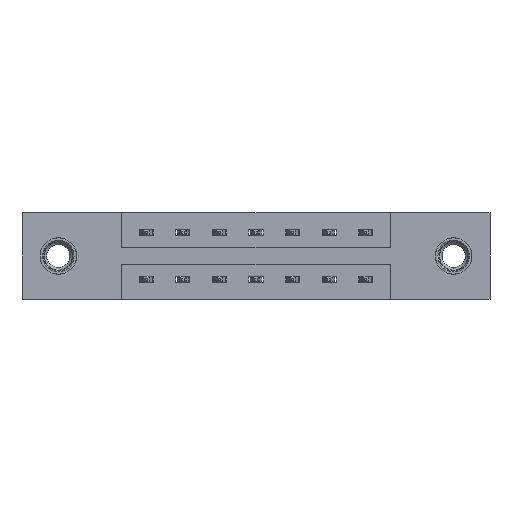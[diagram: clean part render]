
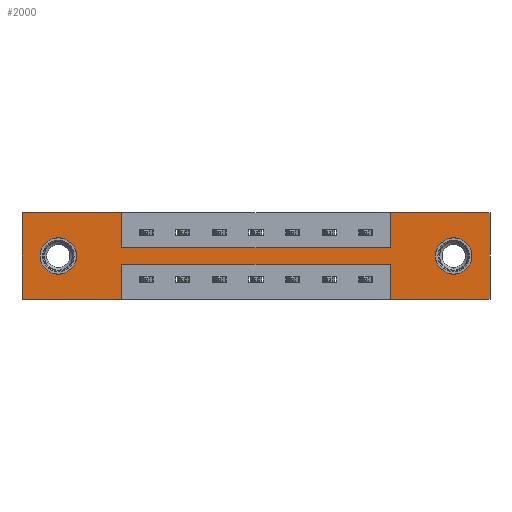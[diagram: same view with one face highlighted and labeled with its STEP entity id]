
A CAD part, front view. The second image highlights one B-rep face of the part: STEP entity #2000.
In plain terms, the highlighted planar face has unit normal (0, -1, 0).
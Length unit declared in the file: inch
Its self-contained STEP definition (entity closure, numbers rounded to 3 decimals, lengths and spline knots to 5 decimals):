
#55 = CIRCLE ( 'NONE', #7593, 0.078 ) ;
#104 = CARTESIAN_POINT ( 'NONE',  ( 1.573, 0., -0.37 ) ) ;
#157 = VECTOR ( 'NONE', #338, 39.37008 ) ;
#312 = DIRECTION ( 'NONE',  ( -1., 0., 0. ) ) ;
#338 = DIRECTION ( 'NONE',  ( 0., 0., -1. ) ) ;
#471 = LINE ( 'NONE', #9917, #2218 ) ;
#537 = CARTESIAN_POINT ( 'NONE',  ( 0., 0., 0. ) ) ;
#622 = VERTEX_POINT ( 'NONE', #3019 ) ;
#650 = DIRECTION ( 'NONE',  ( 0., 1., 0. ) ) ;
#670 = VERTEX_POINT ( 'NONE', #10008 ) ;
#766 = ORIENTED_EDGE ( 'NONE', *, *, #3446, .F. ) ;
#827 = CARTESIAN_POINT ( 'NONE',  ( 0.425, 0., -0.22 ) ) ;
#854 = DIRECTION ( 'NONE',  ( 0., 0., 1. ) ) ;
#955 = VECTOR ( 'NONE', #9980, 39.37008 ) ;
#989 = LINE ( 'NONE', #8020, #9770 ) ;
#1223 = PLANE ( 'NONE',  #6066 ) ;
#1241 = LINE ( 'NONE', #2025, #4396 ) ;
#1275 = LINE ( 'NONE', #104, #6549 ) ;
#1398 = LINE ( 'NONE', #1967, #10052 ) ;
#1524 = DIRECTION ( 'NONE',  ( 0., 1., 0. ) ) ;
#1529 = AXIS2_PLACEMENT_3D ( 'NONE', #5044, #1524, #4934 ) ;
#1532 = VERTEX_POINT ( 'NONE', #7224 ) ;
#1726 = ORIENTED_EDGE ( 'NONE', *, *, #8348, .F. ) ;
#1783 = CIRCLE ( 'NONE', #11081, 0.078 ) ;
#1812 = FACE_BOUND ( 'NONE', #8719, .T. ) ;
#1815 = DIRECTION ( 'NONE',  ( 0., 0., 1. ) ) ;
#1873 = EDGE_CURVE ( 'NONE', #10824, #5733, #471, .T. ) ;
#1967 = CARTESIAN_POINT ( 'NONE',  ( 0.425, 0., -0.22 ) ) ;
#1980 = VECTOR ( 'NONE', #2939, 39.37008 ) ;
#2000 = ADVANCED_FACE ( 'NONE', ( #6968, #1812, #3313 ), #1223, .T. ) ;
#2010 = DIRECTION ( 'NONE',  ( 0., 0., -1. ) ) ;
#2025 = CARTESIAN_POINT ( 'NONE',  ( 0., 0., 0. ) ) ;
#2090 = ORIENTED_EDGE ( 'NONE', *, *, #8855, .F. ) ;
#2108 = CARTESIAN_POINT ( 'NONE',  ( 1.573, 0., -0.15 ) ) ;
#2112 = VERTEX_POINT ( 'NONE', #827 ) ;
#2218 = VECTOR ( 'NONE', #7230, 39.37008 ) ;
#2241 = VERTEX_POINT ( 'NONE', #7441 ) ;
#2256 = CARTESIAN_POINT ( 'NONE',  ( 0.155, 0., -0.185 ) ) ;
#2278 = ORIENTED_EDGE ( 'NONE', *, *, #1873, .F. ) ;
#2280 = DIRECTION ( 'NONE',  ( 0., 0., -1. ) ) ;
#2353 = DIRECTION ( 'NONE',  ( 0., 0., 1. ) ) ;
#2492 = CARTESIAN_POINT ( 'NONE',  ( 0., 0., 0. ) ) ;
#2566 = DIRECTION ( 'NONE',  ( 1., 0., 0. ) ) ;
#2665 = CARTESIAN_POINT ( 'NONE',  ( 0.425, 0., -0.15 ) ) ;
#2847 = ORIENTED_EDGE ( 'NONE', *, *, #11093, .F. ) ;
#2856 = CARTESIAN_POINT ( 'NONE',  ( 0., 0., -0.37 ) ) ;
#2877 = DIRECTION ( 'NONE',  ( 0., 0., -1. ) ) ;
#2923 = DIRECTION ( 'NONE',  ( -1., 0., 0. ) ) ;
#2928 = EDGE_CURVE ( 'NONE', #670, #7029, #5459, .T. ) ;
#2939 = DIRECTION ( 'NONE',  ( 0., 0., -1. ) ) ;
#3000 = ORIENTED_EDGE ( 'NONE', *, *, #4645, .F. ) ;
#3019 = CARTESIAN_POINT ( 'NONE',  ( 0.425, 0., -0.37 ) ) ;
#3028 = EDGE_CURVE ( 'NONE', #10670, #10953, #11077, .T. ) ;
#3039 = AXIS2_PLACEMENT_3D ( 'NONE', #4877, #10363, #854 ) ;
#3173 = VERTEX_POINT ( 'NONE', #9330 ) ;
#3174 = CARTESIAN_POINT ( 'NONE',  ( 1.843, 0., -0.185 ) ) ;
#3216 = DIRECTION ( 'NONE',  ( 0., 0., 1. ) ) ;
#3248 = LINE ( 'NONE', #2492, #7688 ) ;
#3313 = FACE_OUTER_BOUND ( 'NONE', #5036, .T. ) ;
#3354 = CARTESIAN_POINT ( 'NONE',  ( 1.573, 0., 0. ) ) ;
#3416 = ORIENTED_EDGE ( 'NONE', *, *, #3631, .T. ) ;
#3446 = EDGE_CURVE ( 'NONE', #2112, #622, #5840, .T. ) ;
#3631 = EDGE_CURVE ( 'NONE', #10953, #10670, #1783, .T. ) ;
#3747 = ORIENTED_EDGE ( 'NONE', *, *, #2928, .F. ) ;
#4039 = EDGE_CURVE ( 'NONE', #4281, #10824, #8648, .T. ) ;
#4068 = VERTEX_POINT ( 'NONE', #5375 ) ;
#4095 = CARTESIAN_POINT ( 'NONE',  ( 1.843, 0., -0.263 ) ) ;
#4101 = ORIENTED_EDGE ( 'NONE', *, *, #10692, .T. ) ;
#4281 = VERTEX_POINT ( 'NONE', #9925 ) ;
#4396 = VECTOR ( 'NONE', #5483, 39.37008 ) ;
#4645 = EDGE_CURVE ( 'NONE', #4068, #1532, #6584, .T. ) ;
#4877 = CARTESIAN_POINT ( 'NONE',  ( 0.155, 0., -0.185 ) ) ;
#4897 = VECTOR ( 'NONE', #2353, 39.37008 ) ;
#4934 = DIRECTION ( 'NONE',  ( 0., 0., -1. ) ) ;
#4940 = VERTEX_POINT ( 'NONE', #10927 ) ;
#5036 = EDGE_LOOP ( 'NONE', ( #766, #5313, #8299, #7612, #3000, #2090, #1726, #2278, #10695, #2847, #3747, #10406 ) ) ;
#5044 = CARTESIAN_POINT ( 'NONE',  ( 1.843, 0., -0.185 ) ) ;
#5313 = ORIENTED_EDGE ( 'NONE', *, *, #6135, .F. ) ;
#5375 = CARTESIAN_POINT ( 'NONE',  ( 1.998, 0., 0. ) ) ;
#5435 = EDGE_LOOP ( 'NONE', ( #5589, #3416 ) ) ;
#5459 = LINE ( 'NONE', #537, #7866 ) ;
#5483 = DIRECTION ( 'NONE',  ( 1., 0., 0. ) ) ;
#5589 = ORIENTED_EDGE ( 'NONE', *, *, #3028, .T. ) ;
#5645 = DIRECTION ( 'NONE',  ( 0., 0., 1. ) ) ;
#5733 = VERTEX_POINT ( 'NONE', #2108 ) ;
#5840 = LINE ( 'NONE', #8085, #157 ) ;
#5919 = EDGE_CURVE ( 'NONE', #6405, #4940, #1275, .T. ) ;
#5978 = CARTESIAN_POINT ( 'NONE',  ( 1.573, 0., -0.37 ) ) ;
#6066 = AXIS2_PLACEMENT_3D ( 'NONE', #8647, #7202, #2010 ) ;
#6135 = EDGE_CURVE ( 'NONE', #4940, #2112, #1398, .T. ) ;
#6215 = CARTESIAN_POINT ( 'NONE',  ( 0., 0., 0. ) ) ;
#6286 = EDGE_CURVE ( 'NONE', #7742, #2241, #55, .T. ) ;
#6299 = CARTESIAN_POINT ( 'NONE',  ( 0.425, 0., 0. ) ) ;
#6377 = VECTOR ( 'NONE', #2877, 39.37008 ) ;
#6382 = ORIENTED_EDGE ( 'NONE', *, *, #6286, .T. ) ;
#6405 = VERTEX_POINT ( 'NONE', #5978 ) ;
#6549 = VECTOR ( 'NONE', #1815, 39.37008 ) ;
#6584 = LINE ( 'NONE', #10542, #1980 ) ;
#6968 = FACE_BOUND ( 'NONE', #5435, .T. ) ;
#7029 = VERTEX_POINT ( 'NONE', #6215 ) ;
#7202 = DIRECTION ( 'NONE',  ( 0., -1., 0. ) ) ;
#7224 = CARTESIAN_POINT ( 'NONE',  ( 1.998, 0., -0.37 ) ) ;
#7230 = DIRECTION ( 'NONE',  ( 1., 0., 0. ) ) ;
#7338 = CIRCLE ( 'NONE', #3039, 0.078 ) ;
#7441 = CARTESIAN_POINT ( 'NONE',  ( 0.155, 0., -0.263 ) ) ;
#7593 = AXIS2_PLACEMENT_3D ( 'NONE', #2256, #650, #3216 ) ;
#7612 = ORIENTED_EDGE ( 'NONE', *, *, #11122, .F. ) ;
#7688 = VECTOR ( 'NONE', #2566, 39.37008 ) ;
#7742 = VERTEX_POINT ( 'NONE', #10509 ) ;
#7866 = VECTOR ( 'NONE', #5645, 39.37008 ) ;
#8020 = CARTESIAN_POINT ( 'NONE',  ( 0., 0., -0.37 ) ) ;
#8085 = CARTESIAN_POINT ( 'NONE',  ( 0.425, 0., -0.37 ) ) ;
#8299 = ORIENTED_EDGE ( 'NONE', *, *, #5919, .F. ) ;
#8348 = EDGE_CURVE ( 'NONE', #5733, #3173, #9462, .T. ) ;
#8558 = EDGE_CURVE ( 'NONE', #622, #670, #9021, .T. ) ;
#8647 = CARTESIAN_POINT ( 'NONE',  ( 0., 0., -0.37 ) ) ;
#8648 = LINE ( 'NONE', #6299, #6377 ) ;
#8719 = EDGE_LOOP ( 'NONE', ( #6382, #4101 ) ) ;
#8855 = EDGE_CURVE ( 'NONE', #3173, #4068, #3248, .T. ) ;
#9021 = LINE ( 'NONE', #2856, #955 ) ;
#9330 = CARTESIAN_POINT ( 'NONE',  ( 1.573, 0., 0. ) ) ;
#9462 = LINE ( 'NONE', #3354, #4897 ) ;
#9770 = VECTOR ( 'NONE', #2923, 39.37008 ) ;
#9917 = CARTESIAN_POINT ( 'NONE',  ( 0.425, 0., -0.15 ) ) ;
#9925 = CARTESIAN_POINT ( 'NONE',  ( 0.425, 0., 0. ) ) ;
#9939 = DIRECTION ( 'NONE',  ( 0., 1., 0. ) ) ;
#9980 = DIRECTION ( 'NONE',  ( -1., 0., 0. ) ) ;
#10008 = CARTESIAN_POINT ( 'NONE',  ( 0., 0., -0.37 ) ) ;
#10052 = VECTOR ( 'NONE', #312, 39.37008 ) ;
#10323 = CARTESIAN_POINT ( 'NONE',  ( 1.843, 0., -0.107 ) ) ;
#10363 = DIRECTION ( 'NONE',  ( 0., 1., 0. ) ) ;
#10406 = ORIENTED_EDGE ( 'NONE', *, *, #8558, .F. ) ;
#10509 = CARTESIAN_POINT ( 'NONE',  ( 0.155, 0., -0.107 ) ) ;
#10542 = CARTESIAN_POINT ( 'NONE',  ( 1.998, 0., 0. ) ) ;
#10670 = VERTEX_POINT ( 'NONE', #10323 ) ;
#10692 = EDGE_CURVE ( 'NONE', #2241, #7742, #7338, .T. ) ;
#10695 = ORIENTED_EDGE ( 'NONE', *, *, #4039, .F. ) ;
#10824 = VERTEX_POINT ( 'NONE', #2665 ) ;
#10927 = CARTESIAN_POINT ( 'NONE',  ( 1.573, 0., -0.22 ) ) ;
#10953 = VERTEX_POINT ( 'NONE', #4095 ) ;
#11077 = CIRCLE ( 'NONE', #1529, 0.078 ) ;
#11081 = AXIS2_PLACEMENT_3D ( 'NONE', #3174, #9939, #2280 ) ;
#11093 = EDGE_CURVE ( 'NONE', #7029, #4281, #1241, .T. ) ;
#11122 = EDGE_CURVE ( 'NONE', #1532, #6405, #989, .T. ) ;
